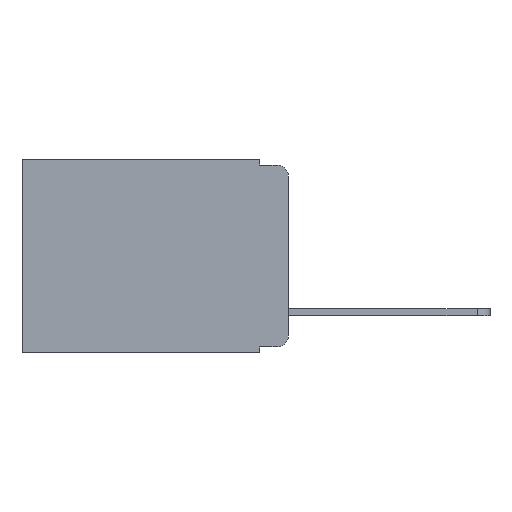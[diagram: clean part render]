
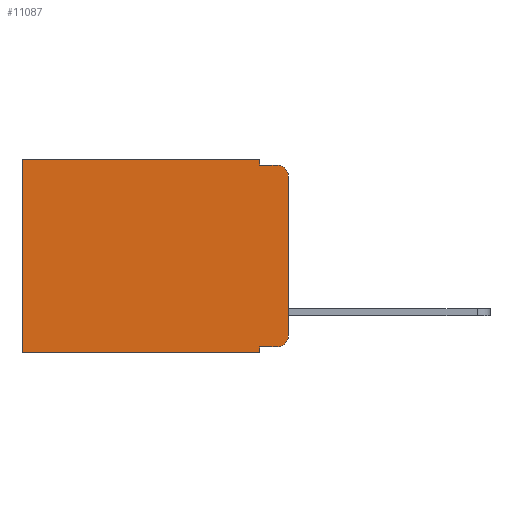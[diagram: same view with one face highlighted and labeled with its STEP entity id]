
A CAD part, left-side view. The second image highlights one B-rep face of the part: STEP entity #11087.
In plain terms, the highlighted planar face has unit normal (-1, 0, 0).
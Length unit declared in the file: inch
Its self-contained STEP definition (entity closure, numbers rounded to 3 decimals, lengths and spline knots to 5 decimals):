
#93 = DIRECTION ( 'NONE',  ( 0., 0., -1. ) ) ;
#121 = CARTESIAN_POINT ( 'NONE',  ( 0.298, 0., -0.343 ) ) ;
#217 = VERTEX_POINT ( 'NONE', #13732 ) ;
#283 = LINE ( 'NONE', #5568, #14221 ) ;
#354 = EDGE_CURVE ( 'NONE', #217, #3455, #2325, .T. ) ;
#445 = CARTESIAN_POINT ( 'NONE',  ( 0.298, 0., 0. ) ) ;
#830 = LINE ( 'NONE', #6205, #6366 ) ;
#862 = CARTESIAN_POINT ( 'NONE',  ( 0.298, 0., -0.03 ) ) ;
#953 = VERTEX_POINT ( 'NONE', #9019 ) ;
#1179 = EDGE_CURVE ( 'NONE', #953, #1734, #4389, .T. ) ;
#1688 = CARTESIAN_POINT ( 'NONE',  ( 0.298, 0.473, 0. ) ) ;
#1694 = ORIENTED_EDGE ( 'NONE', *, *, #5352, .F. ) ;
#1734 = VERTEX_POINT ( 'NONE', #13951 ) ;
#2203 = LINE ( 'NONE', #9772, #7873 ) ;
#2301 = DIRECTION ( 'NONE',  ( 0., 0., -1. ) ) ;
#2325 = LINE ( 'NONE', #121, #11422 ) ;
#2332 = VECTOR ( 'NONE', #12312, 39.37008 ) ;
#2456 = DIRECTION ( 'NONE',  ( -1., 0., 0. ) ) ;
#2462 = CARTESIAN_POINT ( 'NONE',  ( 0.298, 0.02, -0.03 ) ) ;
#2490 = LINE ( 'NONE', #7638, #10935 ) ;
#2660 = AXIS2_PLACEMENT_3D ( 'NONE', #14096, #3149, #12850 ) ;
#2938 = EDGE_CURVE ( 'NONE', #4416, #10969, #9840, .T. ) ;
#3149 = DIRECTION ( 'NONE',  ( -1., 0., 0. ) ) ;
#3201 = CARTESIAN_POINT ( 'NONE',  ( 0.298, 0.473, 0. ) ) ;
#3405 = ORIENTED_EDGE ( 'NONE', *, *, #354, .F. ) ;
#3422 = EDGE_CURVE ( 'NONE', #10659, #953, #9670, .T. ) ;
#3455 = VERTEX_POINT ( 'NONE', #13931 ) ;
#4389 = CIRCLE ( 'NONE', #2660, 0.02 ) ;
#4416 = VERTEX_POINT ( 'NONE', #862 ) ;
#4446 = ORIENTED_EDGE ( 'NONE', *, *, #12866, .T. ) ;
#4728 = DIRECTION ( 'NONE',  ( 1., 0., 0. ) ) ;
#5054 = DIRECTION ( 'NONE',  ( 0., -1., 0. ) ) ;
#5139 = EDGE_CURVE ( 'NONE', #4416, #1734, #5256, .T. ) ;
#5238 = EDGE_CURVE ( 'NONE', #10838, #3455, #10087, .T. ) ;
#5256 = LINE ( 'NONE', #445, #2332 ) ;
#5352 = EDGE_CURVE ( 'NONE', #10659, #217, #2490, .T. ) ;
#5568 = CARTESIAN_POINT ( 'NONE',  ( 0.298, 0., 0. ) ) ;
#5822 = VERTEX_POINT ( 'NONE', #6497 ) ;
#6205 = CARTESIAN_POINT ( 'NONE',  ( 0.298, 0.051, 0. ) ) ;
#6366 = VECTOR ( 'NONE', #7307, 39.37008 ) ;
#6497 = CARTESIAN_POINT ( 'NONE',  ( 0.298, 0.051, -0.01 ) ) ;
#6667 = DIRECTION ( 'NONE',  ( 0., 1., 0. ) ) ;
#6691 = EDGE_LOOP ( 'NONE', ( #11821, #7846, #7514, #12468, #4446, #6980, #3405, #1694, #11138, #12989 ) ) ;
#6702 = DIRECTION ( 'NONE',  ( 0., 0., -1. ) ) ;
#6897 = DIRECTION ( 'NONE',  ( 0., 1., 0. ) ) ;
#6980 = ORIENTED_EDGE ( 'NONE', *, *, #5238, .T. ) ;
#7307 = DIRECTION ( 'NONE',  ( 0., 0., -1. ) ) ;
#7514 = ORIENTED_EDGE ( 'NONE', *, *, #9565, .F. ) ;
#7638 = CARTESIAN_POINT ( 'NONE',  ( 0.298, 0.051, 0. ) ) ;
#7846 = ORIENTED_EDGE ( 'NONE', *, *, #2938, .T. ) ;
#7873 = VECTOR ( 'NONE', #8659, 39.37008 ) ;
#8373 = AXIS2_PLACEMENT_3D ( 'NONE', #2462, #2456, #93 ) ;
#8659 = DIRECTION ( 'NONE',  ( 0., -1., 0. ) ) ;
#9019 = CARTESIAN_POINT ( 'NONE',  ( 0.298, 0.02, -0.333 ) ) ;
#9565 = EDGE_CURVE ( 'NONE', #5822, #10969, #2203, .T. ) ;
#9640 = CARTESIAN_POINT ( 'NONE',  ( 0.298, 0.051, -0.333 ) ) ;
#9670 = LINE ( 'NONE', #9640, #12218 ) ;
#9744 = VECTOR ( 'NONE', #2301, 39.37008 ) ;
#9772 = CARTESIAN_POINT ( 'NONE',  ( 0.298, 0.051, -0.01 ) ) ;
#9840 = CIRCLE ( 'NONE', #8373, 0.02 ) ;
#10087 = LINE ( 'NONE', #1688, #9744 ) ;
#10591 = CARTESIAN_POINT ( 'NONE',  ( 0.298, 0.051, 0. ) ) ;
#10659 = VERTEX_POINT ( 'NONE', #12721 ) ;
#10684 = VERTEX_POINT ( 'NONE', #10591 ) ;
#10741 = AXIS2_PLACEMENT_3D ( 'NONE', #13412, #4728, #12381 ) ;
#10838 = VERTEX_POINT ( 'NONE', #3201 ) ;
#10935 = VECTOR ( 'NONE', #6702, 39.37008 ) ;
#10969 = VERTEX_POINT ( 'NONE', #11113 ) ;
#11087 = ADVANCED_FACE ( 'NONE', ( #13240 ), #11289, .F. ) ;
#11113 = CARTESIAN_POINT ( 'NONE',  ( 0.298, 0.02, -0.01 ) ) ;
#11138 = ORIENTED_EDGE ( 'NONE', *, *, #3422, .T. ) ;
#11289 = PLANE ( 'NONE',  #10741 ) ;
#11422 = VECTOR ( 'NONE', #6897, 39.37008 ) ;
#11821 = ORIENTED_EDGE ( 'NONE', *, *, #5139, .F. ) ;
#11964 = EDGE_CURVE ( 'NONE', #10684, #5822, #830, .T. ) ;
#12218 = VECTOR ( 'NONE', #5054, 39.37008 ) ;
#12312 = DIRECTION ( 'NONE',  ( 0., 0., -1. ) ) ;
#12381 = DIRECTION ( 'NONE',  ( 0., 0., -1. ) ) ;
#12468 = ORIENTED_EDGE ( 'NONE', *, *, #11964, .F. ) ;
#12721 = CARTESIAN_POINT ( 'NONE',  ( 0.298, 0.051, -0.333 ) ) ;
#12850 = DIRECTION ( 'NONE',  ( 0., 0., -1. ) ) ;
#12866 = EDGE_CURVE ( 'NONE', #10684, #10838, #283, .T. ) ;
#12989 = ORIENTED_EDGE ( 'NONE', *, *, #1179, .T. ) ;
#13240 = FACE_OUTER_BOUND ( 'NONE', #6691, .T. ) ;
#13412 = CARTESIAN_POINT ( 'NONE',  ( 0.298, 0., 0. ) ) ;
#13732 = CARTESIAN_POINT ( 'NONE',  ( 0.298, 0.051, -0.343 ) ) ;
#13931 = CARTESIAN_POINT ( 'NONE',  ( 0.298, 0.473, -0.343 ) ) ;
#13951 = CARTESIAN_POINT ( 'NONE',  ( 0.298, 0., -0.313 ) ) ;
#14096 = CARTESIAN_POINT ( 'NONE',  ( 0.298, 0.02, -0.313 ) ) ;
#14221 = VECTOR ( 'NONE', #6667, 39.37008 ) ;
